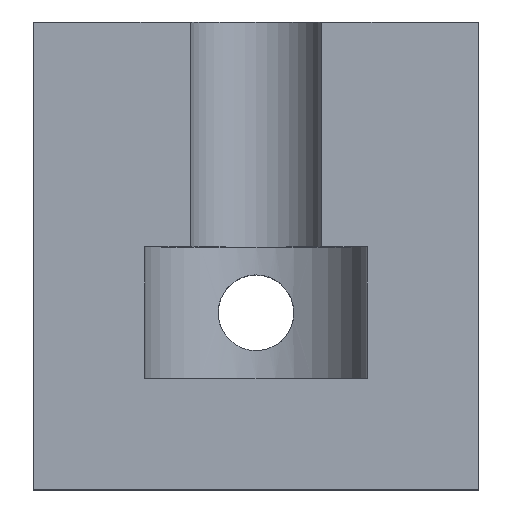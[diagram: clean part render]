
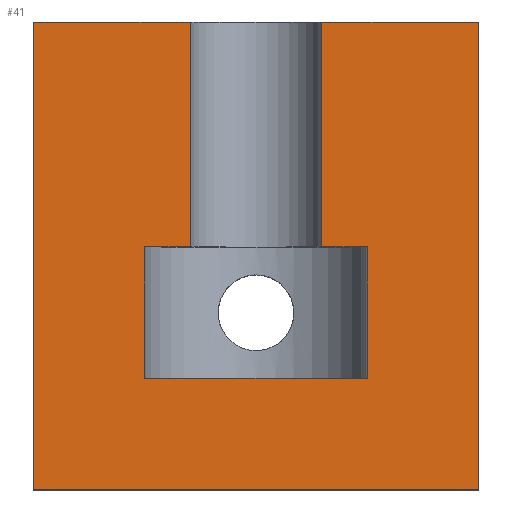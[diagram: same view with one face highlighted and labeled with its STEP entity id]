
A CAD part, top view. The second image highlights one B-rep face of the part: STEP entity #41.
In plain terms, the highlighted planar face has unit normal (0, 0, 1).
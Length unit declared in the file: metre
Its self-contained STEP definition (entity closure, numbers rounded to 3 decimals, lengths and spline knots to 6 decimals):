
#41 = ADVANCED_FACE( '', ( #83 ), #84, .T. );
#83 = FACE_OUTER_BOUND( '', #126, .T. );
#84 = PLANE( '', #127 );
#126 = EDGE_LOOP( '', ( #176, #177, #178, #179, #180, #181, #182, #183, #184, #185, #186, #187 ) );
#127 = AXIS2_PLACEMENT_3D( '', #188, #189, #190 );
#176 = ORIENTED_EDGE( '', *, *, #263, .F. );
#177 = ORIENTED_EDGE( '', *, *, #250, .T. );
#178 = ORIENTED_EDGE( '', *, *, #264, .F. );
#179 = ORIENTED_EDGE( '', *, *, #265, .F. );
#180 = ORIENTED_EDGE( '', *, *, #266, .F. );
#181 = ORIENTED_EDGE( '', *, *, #255, .T. );
#182 = ORIENTED_EDGE( '', *, *, #267, .T. );
#183 = ORIENTED_EDGE( '', *, *, #268, .F. );
#184 = ORIENTED_EDGE( '', *, *, #269, .T. );
#185 = ORIENTED_EDGE( '', *, *, #252, .T. );
#186 = ORIENTED_EDGE( '', *, *, #270, .T. );
#187 = ORIENTED_EDGE( '', *, *, #261, .F. );
#188 = CARTESIAN_POINT( '', ( 0.01, 0.008, 0.01 ) );
#189 = DIRECTION( '', ( 0., 0., 1. ) );
#190 = DIRECTION( '', ( 1., 0., 0. ) );
#250 = EDGE_CURVE( '', #287, #288, #289, .T. );
#252 = EDGE_CURVE( '', #292, #290, #293, .T. );
#255 = EDGE_CURVE( '', #296, #297, #298, .T. );
#261 = EDGE_CURVE( '', #305, #306, #308, .T. );
#263 = EDGE_CURVE( '', #287, #305, #310, .T. );
#264 = EDGE_CURVE( '', #311, #288, #312, .T. );
#265 = EDGE_CURVE( '', #313, #311, #314, .T. );
#266 = EDGE_CURVE( '', #296, #313, #315, .T. );
#267 = EDGE_CURVE( '', #297, #316, #317, .T. );
#268 = EDGE_CURVE( '', #318, #316, #319, .T. );
#269 = EDGE_CURVE( '', #318, #292, #320, .T. );
#270 = EDGE_CURVE( '', #290, #306, #321, .T. );
#287 = VERTEX_POINT( '', #342 );
#288 = VERTEX_POINT( '', #343 );
#289 = LINE( '', #344, #345 );
#290 = VERTEX_POINT( '', #346 );
#292 = VERTEX_POINT( '', #348 );
#293 = LINE( '', #349, #350 );
#296 = VERTEX_POINT( '', #353 );
#297 = VERTEX_POINT( '', #354 );
#298 = LINE( '', #355, #356 );
#305 = VERTEX_POINT( '', #366 );
#306 = VERTEX_POINT( '', #367 );
#308 = LINE( '', #369, #370 );
#310 = LINE( '', #372, #373 );
#311 = VERTEX_POINT( '', #374 );
#312 = LINE( '', #375, #376 );
#313 = VERTEX_POINT( '', #377 );
#314 = LINE( '', #378, #379 );
#315 = LINE( '', #380, #381 );
#316 = VERTEX_POINT( '', #382 );
#317 = LINE( '', #383, #384 );
#318 = VERTEX_POINT( '', #385 );
#319 = LINE( '', #386, #387 );
#320 = LINE( '', #388, #389 );
#321 = LINE( '', #390, #391 );
#342 = CARTESIAN_POINT( '', ( 0.005, 0.0059, 0.01 ) );
#343 = CARTESIAN_POINT( '', ( 0.00705, 0.0059, 0.01 ) );
#344 = CARTESIAN_POINT( '', ( 0.01, 0.0059, 0.01 ) );
#345 = VECTOR( '', #471, 1. );
#346 = CARTESIAN_POINT( '', ( 0.015, 0.0059, 0.01 ) );
#348 = CARTESIAN_POINT( '', ( 0.01295, 0.0059, 0.01 ) );
#349 = CARTESIAN_POINT( '', ( 0.01, 0.0059, 0.01 ) );
#350 = VECTOR( '', #475, 1. );
#353 = CARTESIAN_POINT( '', ( 0., -0.005, 0.01 ) );
#354 = CARTESIAN_POINT( '', ( 0.02, -0.005, 0.01 ) );
#355 = CARTESIAN_POINT( '', ( 0.01, -0.005, 0.01 ) );
#356 = VECTOR( '', #479, 1. );
#366 = CARTESIAN_POINT( '', ( 0.005, 0., 0.01 ) );
#367 = CARTESIAN_POINT( '', ( 0.015, 0., 0.01 ) );
#369 = CARTESIAN_POINT( '', ( 0.01, 0., 0.01 ) );
#370 = VECTOR( '', #486, 1. );
#372 = CARTESIAN_POINT( '', ( 0.005, 0.0059, 0.01 ) );
#373 = VECTOR( '', #487, 1. );
#374 = CARTESIAN_POINT( '', ( 0.00705, 0.016, 0.01 ) );
#375 = CARTESIAN_POINT( '', ( 0.00705, 0.016002, 0.01 ) );
#376 = VECTOR( '', #488, 1. );
#377 = CARTESIAN_POINT( '', ( 0., 0.016, 0.01 ) );
#378 = CARTESIAN_POINT( '', ( 0.01, 0.016, 0.01 ) );
#379 = VECTOR( '', #489, 1. );
#380 = CARTESIAN_POINT( '', ( 0., 0.008, 0.01 ) );
#381 = VECTOR( '', #490, 1. );
#382 = CARTESIAN_POINT( '', ( 0.02, 0.016, 0.01 ) );
#383 = CARTESIAN_POINT( '', ( 0.02, 0.008, 0.01 ) );
#384 = VECTOR( '', #491, 1. );
#385 = CARTESIAN_POINT( '', ( 0.01295, 0.016, 0.01 ) );
#386 = CARTESIAN_POINT( '', ( 0.01, 0.016, 0.01 ) );
#387 = VECTOR( '', #492, 1. );
#388 = CARTESIAN_POINT( '', ( 0.01295, 0.016002, 0.01 ) );
#389 = VECTOR( '', #493, 1. );
#390 = CARTESIAN_POINT( '', ( 0.015, 0.0059, 0.01 ) );
#391 = VECTOR( '', #494, 1. );
#471 = DIRECTION( '', ( 1., 0., 0. ) );
#475 = DIRECTION( '', ( 1., 0., 0. ) );
#479 = DIRECTION( '', ( 1., 0., 0. ) );
#486 = DIRECTION( '', ( 1., 0., 0. ) );
#487 = DIRECTION( '', ( 0., -1., 0. ) );
#488 = DIRECTION( '', ( 0., -1., 0. ) );
#489 = DIRECTION( '', ( 1., 0., 0. ) );
#490 = DIRECTION( '', ( 0., 1., 0. ) );
#491 = DIRECTION( '', ( 0., 1., 0. ) );
#492 = DIRECTION( '', ( 1., 0., 0. ) );
#493 = DIRECTION( '', ( 0., -1., 0. ) );
#494 = DIRECTION( '', ( 0., -1., 0. ) );
